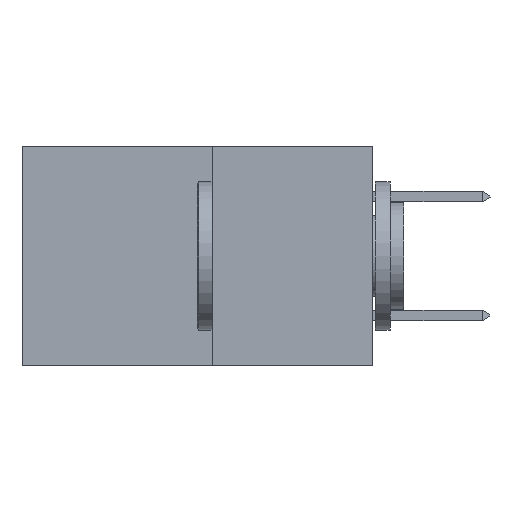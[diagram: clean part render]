
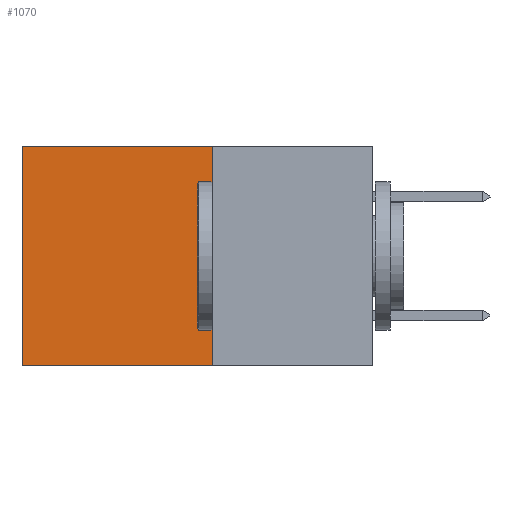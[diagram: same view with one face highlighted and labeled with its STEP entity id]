
A CAD part, left-side view. The second image highlights one B-rep face of the part: STEP entity #1070.
In plain terms, the highlighted planar face has unit normal (-1, 0, 0).
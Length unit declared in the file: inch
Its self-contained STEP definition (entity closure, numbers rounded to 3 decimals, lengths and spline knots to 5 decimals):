
#101 = CARTESIAN_POINT ( 'NONE',  ( 0.277, 0.59, 0. ) ) ;
#104 = VERTEX_POINT ( 'NONE', #8418 ) ;
#107 = EDGE_CURVE ( 'NONE', #9368, #104, #9710, .T. ) ;
#999 = VECTOR ( 'NONE', #5685, 39.37008 ) ;
#1070 = ADVANCED_FACE ( 'NONE', ( #6252 ), #3394, .F. ) ;
#1738 = CARTESIAN_POINT ( 'NONE',  ( 0.277, 0.27, -0.37 ) ) ;
#2454 = ORIENTED_EDGE ( 'NONE', *, *, #7089, .T. ) ;
#2643 = VECTOR ( 'NONE', #7004, 39.37008 ) ;
#3145 = CARTESIAN_POINT ( 'NONE',  ( 0.277, 0.59, -0.37 ) ) ;
#3227 = DIRECTION ( 'NONE',  ( 1., 0., 0. ) ) ;
#3345 = EDGE_LOOP ( 'NONE', ( #2454, #5920, #7473, #8961 ) ) ;
#3394 = PLANE ( 'NONE',  #4413 ) ;
#4005 = DIRECTION ( 'NONE',  ( 0., 0., -1. ) ) ;
#4233 = EDGE_CURVE ( 'NONE', #9368, #9522, #8236, .T. ) ;
#4373 = CARTESIAN_POINT ( 'NONE',  ( 0.277, 0.27, -0.37 ) ) ;
#4413 = AXIS2_PLACEMENT_3D ( 'NONE', #1738, #3227, #4005 ) ;
#4572 = DIRECTION ( 'NONE',  ( 0., 0., -1. ) ) ;
#4827 = CARTESIAN_POINT ( 'NONE',  ( 0.277, 0.27, 0. ) ) ;
#5685 = DIRECTION ( 'NONE',  ( 0., 1., 0. ) ) ;
#5911 = LINE ( 'NONE', #3145, #9731 ) ;
#5920 = ORIENTED_EDGE ( 'NONE', *, *, #10017, .F. ) ;
#6173 = CARTESIAN_POINT ( 'NONE',  ( 0.277, 0.27, -0.37 ) ) ;
#6252 = FACE_OUTER_BOUND ( 'NONE', #3345, .T. ) ;
#6744 = CARTESIAN_POINT ( 'NONE',  ( 0.277, 0.27, 0. ) ) ;
#7004 = DIRECTION ( 'NONE',  ( 0., 1., 0. ) ) ;
#7089 = EDGE_CURVE ( 'NONE', #9522, #10580, #5911, .T. ) ;
#7473 = ORIENTED_EDGE ( 'NONE', *, *, #107, .F. ) ;
#7760 = VECTOR ( 'NONE', #4572, 39.37008 ) ;
#8236 = LINE ( 'NONE', #4827, #999 ) ;
#8418 = CARTESIAN_POINT ( 'NONE',  ( 0.277, 0.27, -0.37 ) ) ;
#8769 = CARTESIAN_POINT ( 'NONE',  ( 0.277, 0.59, -0.37 ) ) ;
#8961 = ORIENTED_EDGE ( 'NONE', *, *, #4233, .T. ) ;
#9368 = VERTEX_POINT ( 'NONE', #6744 ) ;
#9522 = VERTEX_POINT ( 'NONE', #101 ) ;
#9710 = LINE ( 'NONE', #4373, #7760 ) ;
#9731 = VECTOR ( 'NONE', #9736, 39.37008 ) ;
#9736 = DIRECTION ( 'NONE',  ( 0., 0., -1. ) ) ;
#10017 = EDGE_CURVE ( 'NONE', #104, #10580, #11202, .T. ) ;
#10580 = VERTEX_POINT ( 'NONE', #8769 ) ;
#11202 = LINE ( 'NONE', #6173, #2643 ) ;
